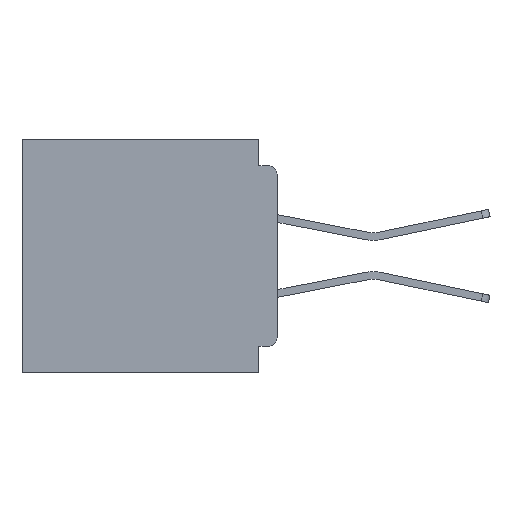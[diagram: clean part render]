
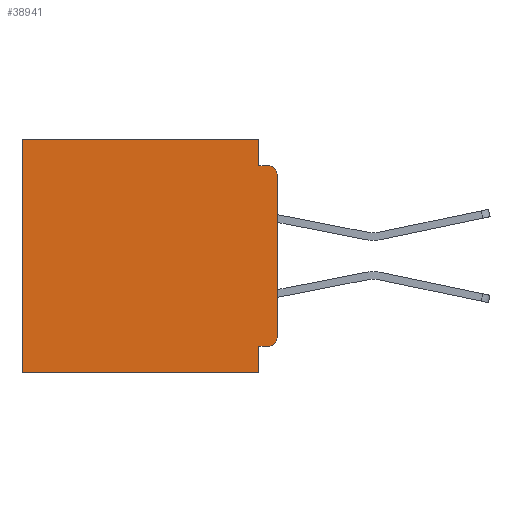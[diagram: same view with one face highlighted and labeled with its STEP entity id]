
A CAD part, left-side view. The second image highlights one B-rep face of the part: STEP entity #38941.
In plain terms, the highlighted planar face has unit normal (-1, 0, 0).
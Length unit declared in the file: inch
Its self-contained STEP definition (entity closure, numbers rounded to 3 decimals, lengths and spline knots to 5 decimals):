
#213 = AXIS2_PLACEMENT_3D ( 'NONE', #21715, #48487, #25592 ) ;
#1168 = CARTESIAN_POINT ( 'NONE',  ( 0.3, 0.031, -0.355 ) ) ;
#1823 = EDGE_CURVE ( 'NONE', #24492, #35299, #8855, .T. ) ;
#1872 = CIRCLE ( 'NONE', #13677, 0.015 ) ;
#1967 = AXIS2_PLACEMENT_3D ( 'NONE', #25448, #2442, #29307 ) ;
#2442 = DIRECTION ( 'NONE',  ( 1., 0., 0. ) ) ;
#2792 = EDGE_CURVE ( 'NONE', #17110, #33954, #48450, .T. ) ;
#2874 = EDGE_CURVE ( 'NONE', #4728, #36404, #23315, .T. ) ;
#3108 = DIRECTION ( 'NONE',  ( 0., 0., -1. ) ) ;
#3318 = CARTESIAN_POINT ( 'NONE',  ( 0.3, 0.437, -0.4 ) ) ;
#4121 = VECTOR ( 'NONE', #45886, 39.37008 ) ;
#4232 = FACE_OUTER_BOUND ( 'NONE', #39445, .T. ) ;
#4728 = VERTEX_POINT ( 'NONE', #31656 ) ;
#4785 = VECTOR ( 'NONE', #16735, 39.37008 ) ;
#6315 = CARTESIAN_POINT ( 'NONE',  ( 0.3, 0.031, 0. ) ) ;
#6742 = ORIENTED_EDGE ( 'NONE', *, *, #32990, .F. ) ;
#7644 = ORIENTED_EDGE ( 'NONE', *, *, #2874, .F. ) ;
#7762 = VECTOR ( 'NONE', #22276, 39.37008 ) ;
#8131 = CARTESIAN_POINT ( 'NONE',  ( 0.3, 0., -0.06 ) ) ;
#8855 = LINE ( 'NONE', #39643, #19064 ) ;
#9175 = CARTESIAN_POINT ( 'NONE',  ( 0.3, 0.015, -0.06 ) ) ;
#12817 = DIRECTION ( 'NONE',  ( 0., 0., -1. ) ) ;
#12993 = DIRECTION ( 'NONE',  ( 0., 0., -1. ) ) ;
#13057 = VECTOR ( 'NONE', #17679, 39.37008 ) ;
#13677 = AXIS2_PLACEMENT_3D ( 'NONE', #9175, #36027, #12993 ) ;
#14547 = ORIENTED_EDGE ( 'NONE', *, *, #36775, .F. ) ;
#14957 = LINE ( 'NONE', #39780, #4785 ) ;
#15025 = CARTESIAN_POINT ( 'NONE',  ( 0.3, 0.031, 0. ) ) ;
#15483 = LINE ( 'NONE', #42094, #4121 ) ;
#16091 = ORIENTED_EDGE ( 'NONE', *, *, #44513, .T. ) ;
#16607 = CARTESIAN_POINT ( 'NONE',  ( 0.3, 0., -0.34 ) ) ;
#16670 = VECTOR ( 'NONE', #3108, 39.37008 ) ;
#16735 = DIRECTION ( 'NONE',  ( 0., -1., 0. ) ) ;
#16796 = VERTEX_POINT ( 'NONE', #6315 ) ;
#17110 = VERTEX_POINT ( 'NONE', #8131 ) ;
#17679 = DIRECTION ( 'NONE',  ( 0., 1., 0. ) ) ;
#18002 = CARTESIAN_POINT ( 'NONE',  ( 0.3, 0.031, -0.4 ) ) ;
#18395 = CARTESIAN_POINT ( 'NONE',  ( 0.3, 0.437, 0. ) ) ;
#18509 = EDGE_CURVE ( 'NONE', #36404, #24492, #19854, .T. ) ;
#18901 = DIRECTION ( 'NONE',  ( 0., 0., -1. ) ) ;
#19064 = VECTOR ( 'NONE', #32739, 39.37008 ) ;
#19854 = LINE ( 'NONE', #20229, #28912 ) ;
#20229 = CARTESIAN_POINT ( 'NONE',  ( 0.3, 0.031, -0.4 ) ) ;
#21099 = VERTEX_POINT ( 'NONE', #18395 ) ;
#21318 = VERTEX_POINT ( 'NONE', #46338 ) ;
#21715 = CARTESIAN_POINT ( 'NONE',  ( 0.3, 0.015, -0.34 ) ) ;
#21938 = ORIENTED_EDGE ( 'NONE', *, *, #27141, .T. ) ;
#22276 = DIRECTION ( 'NONE',  ( 0., 0., -1. ) ) ;
#23315 = LINE ( 'NONE', #36319, #13057 ) ;
#23799 = VERTEX_POINT ( 'NONE', #36568 ) ;
#24473 = EDGE_CURVE ( 'NONE', #4728, #33954, #49536, .T. ) ;
#24492 = VERTEX_POINT ( 'NONE', #18002 ) ;
#25448 = CARTESIAN_POINT ( 'NONE',  ( 0.3, 0., -0.4 ) ) ;
#25592 = DIRECTION ( 'NONE',  ( 0., 0., -1. ) ) ;
#27141 = EDGE_CURVE ( 'NONE', #21099, #35299, #47295, .T. ) ;
#28912 = VECTOR ( 'NONE', #12817, 39.37008 ) ;
#29274 = CARTESIAN_POINT ( 'NONE',  ( 0.3, 0., -0.4 ) ) ;
#29307 = DIRECTION ( 'NONE',  ( 0., 0., -1. ) ) ;
#31656 = CARTESIAN_POINT ( 'NONE',  ( 0.3, 0.015, -0.355 ) ) ;
#32681 = VECTOR ( 'NONE', #18901, 39.37008 ) ;
#32739 = DIRECTION ( 'NONE',  ( 0., 1., 0. ) ) ;
#32880 = ORIENTED_EDGE ( 'NONE', *, *, #24473, .T. ) ;
#32990 = EDGE_CURVE ( 'NONE', #21318, #23799, #14957, .T. ) ;
#33511 = ORIENTED_EDGE ( 'NONE', *, *, #1823, .F. ) ;
#33890 = LINE ( 'NONE', #15025, #32681 ) ;
#33954 = VERTEX_POINT ( 'NONE', #16607 ) ;
#35299 = VERTEX_POINT ( 'NONE', #40887 ) ;
#36027 = DIRECTION ( 'NONE',  ( -1., 0., 0. ) ) ;
#36319 = CARTESIAN_POINT ( 'NONE',  ( 0.3, 0., -0.355 ) ) ;
#36404 = VERTEX_POINT ( 'NONE', #1168 ) ;
#36568 = CARTESIAN_POINT ( 'NONE',  ( 0.3, 0.015, -0.045 ) ) ;
#36775 = EDGE_CURVE ( 'NONE', #16796, #21318, #33890, .T. ) ;
#38941 = ADVANCED_FACE ( 'NONE', ( #4232 ), #44523, .F. ) ;
#39445 = EDGE_LOOP ( 'NONE', ( #42479, #16091, #6742, #14547, #46377, #21938, #33511, #41264, #7644, #32880 ) ) ;
#39643 = CARTESIAN_POINT ( 'NONE',  ( 0.3, 0., -0.4 ) ) ;
#39780 = CARTESIAN_POINT ( 'NONE',  ( 0.3, 0., -0.045 ) ) ;
#40291 = EDGE_CURVE ( 'NONE', #16796, #21099, #15483, .T. ) ;
#40887 = CARTESIAN_POINT ( 'NONE',  ( 0.3, 0.437, -0.4 ) ) ;
#41264 = ORIENTED_EDGE ( 'NONE', *, *, #18509, .F. ) ;
#42094 = CARTESIAN_POINT ( 'NONE',  ( 0.3, 0., 0. ) ) ;
#42479 = ORIENTED_EDGE ( 'NONE', *, *, #2792, .F. ) ;
#44513 = EDGE_CURVE ( 'NONE', #17110, #23799, #1872, .T. ) ;
#44523 = PLANE ( 'NONE',  #1967 ) ;
#45886 = DIRECTION ( 'NONE',  ( 0., 1., 0. ) ) ;
#46338 = CARTESIAN_POINT ( 'NONE',  ( 0.3, 0.031, -0.045 ) ) ;
#46377 = ORIENTED_EDGE ( 'NONE', *, *, #40291, .T. ) ;
#47295 = LINE ( 'NONE', #3318, #7762 ) ;
#48450 = LINE ( 'NONE', #29274, #16670 ) ;
#48487 = DIRECTION ( 'NONE',  ( -1., 0., 0. ) ) ;
#49536 = CIRCLE ( 'NONE', #213, 0.015 ) ;
